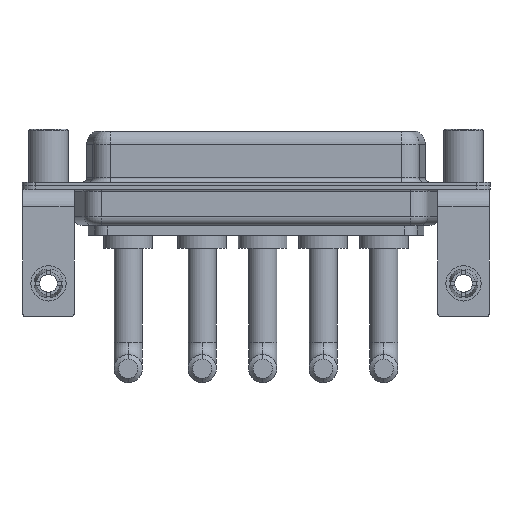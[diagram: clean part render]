
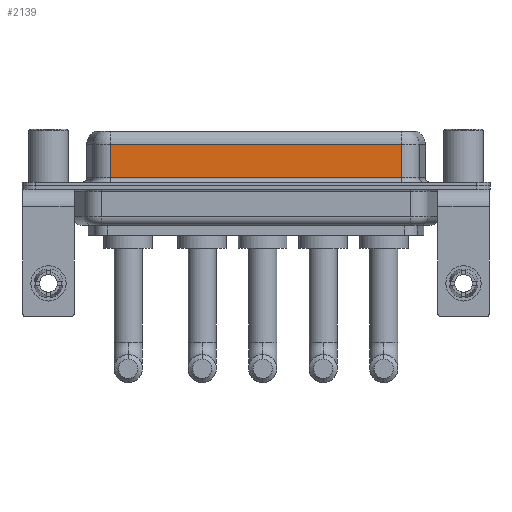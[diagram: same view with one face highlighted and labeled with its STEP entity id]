
A CAD part, front view. The second image highlights one B-rep face of the part: STEP entity #2139.
In plain terms, the highlighted planar face has unit normal (0, -1, 0).
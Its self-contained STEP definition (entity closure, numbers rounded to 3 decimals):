
#427 = VECTOR ( 'NONE', #9556, 1000. ) ;
#1257 = DIRECTION ( 'NONE',  ( 0., 0., -1. ) ) ;
#1727 = ORIENTED_EDGE ( 'NONE', *, *, #7562, .T. ) ;
#1892 = CARTESIAN_POINT ( 'NONE',  ( 40.037, -3.95, 6.4 ) ) ;
#2139 = ADVANCED_FACE ( 'NONE', ( #5722 ), #10941, .F. ) ;
#3420 = LINE ( 'NONE', #8282, #12713 ) ;
#4335 = LINE ( 'NONE', #1892, #427 ) ;
#4393 = CARTESIAN_POINT ( 'NONE',  ( 40.037, -3.95, 0.9 ) ) ;
#4437 = DIRECTION ( 'NONE',  ( 0., 1., 0. ) ) ;
#4447 = VERTEX_POINT ( 'NONE', #4393 ) ;
#4653 = AXIS2_PLACEMENT_3D ( 'NONE', #16159, #4437, #9658 ) ;
#4695 = DIRECTION ( 'NONE',  ( -1., 0., 0. ) ) ;
#5722 = FACE_OUTER_BOUND ( 'NONE', #16551, .T. ) ;
#6309 = ORIENTED_EDGE ( 'NONE', *, *, #7747, .T. ) ;
#6547 = CARTESIAN_POINT ( 'NONE',  ( 40.037, -3.95, 4.65 ) ) ;
#6970 = VECTOR ( 'NONE', #1257, 1000. ) ;
#7562 = EDGE_CURVE ( 'NONE', #16130, #12705, #14216, .T. ) ;
#7721 = CARTESIAN_POINT ( 'NONE',  ( 7.013, -3.95, 6.4 ) ) ;
#7747 = EDGE_CURVE ( 'NONE', #12552, #16130, #3420, .T. ) ;
#8022 = CARTESIAN_POINT ( 'NONE',  ( 40.037, -3.95, 0.9 ) ) ;
#8191 = EDGE_CURVE ( 'NONE', #12705, #4447, #10517, .T. ) ;
#8282 = CARTESIAN_POINT ( 'NONE',  ( 40.037, -3.95, 4.65 ) ) ;
#8363 = EDGE_CURVE ( 'NONE', #12552, #4447, #4335, .T. ) ;
#8472 = CARTESIAN_POINT ( 'NONE',  ( 7.013, -3.95, 0.9 ) ) ;
#8856 = VECTOR ( 'NONE', #14524, 1000. ) ;
#9556 = DIRECTION ( 'NONE',  ( 0., 0., -1. ) ) ;
#9658 = DIRECTION ( 'NONE',  ( 0., 0., 1. ) ) ;
#9756 = ORIENTED_EDGE ( 'NONE', *, *, #8363, .F. ) ;
#10517 = LINE ( 'NONE', #8022, #8856 ) ;
#10941 = PLANE ( 'NONE',  #4653 ) ;
#12552 = VERTEX_POINT ( 'NONE', #6547 ) ;
#12705 = VERTEX_POINT ( 'NONE', #8472 ) ;
#12713 = VECTOR ( 'NONE', #4695, 1000. ) ;
#14216 = LINE ( 'NONE', #7721, #6970 ) ;
#14524 = DIRECTION ( 'NONE',  ( 1., 0., 0. ) ) ;
#16090 = ORIENTED_EDGE ( 'NONE', *, *, #8191, .T. ) ;
#16130 = VERTEX_POINT ( 'NONE', #16279 ) ;
#16159 = CARTESIAN_POINT ( 'NONE',  ( 40.037, -3.95, 6.4 ) ) ;
#16279 = CARTESIAN_POINT ( 'NONE',  ( 7.013, -3.95, 4.65 ) ) ;
#16551 = EDGE_LOOP ( 'NONE', ( #9756, #6309, #1727, #16090 ) ) ;
